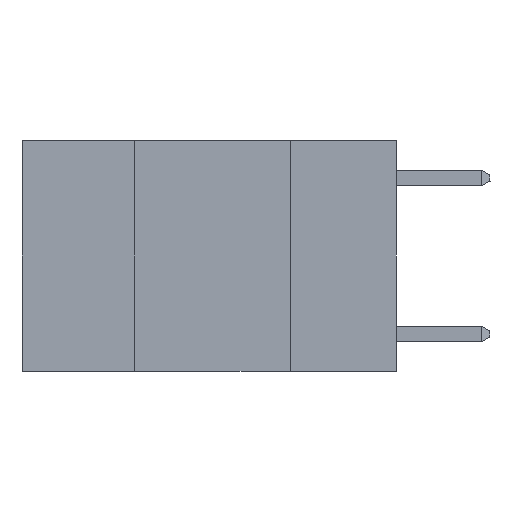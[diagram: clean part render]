
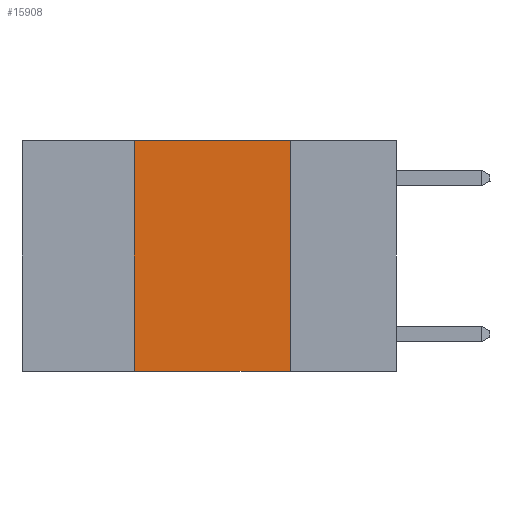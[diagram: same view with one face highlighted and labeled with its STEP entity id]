
A CAD part, left-side view. The second image highlights one B-rep face of the part: STEP entity #15908.
In plain terms, the highlighted planar face has unit normal (-1, 0, 0).
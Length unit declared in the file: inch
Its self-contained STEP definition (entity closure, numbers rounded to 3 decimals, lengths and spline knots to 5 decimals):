
#87 = CARTESIAN_POINT ( 'NONE',  ( 0., 0.42, 0. ) ) ;
#416 = LINE ( 'NONE', #87, #13189 ) ;
#472 = PLANE ( 'NONE',  #19026 ) ;
#810 = EDGE_CURVE ( 'NONE', #15724, #10061, #7259, .T. ) ;
#1289 = VECTOR ( 'NONE', #18226, 39.37008 ) ;
#1603 = CARTESIAN_POINT ( 'NONE',  ( 0., 0.6, 0. ) ) ;
#2174 = DIRECTION ( 'NONE',  ( 1., 0., 0. ) ) ;
#2742 = ORIENTED_EDGE ( 'NONE', *, *, #810, .F. ) ;
#3171 = EDGE_CURVE ( 'NONE', #3308, #10061, #6075, .T. ) ;
#3308 = VERTEX_POINT ( 'NONE', #15059 ) ;
#3775 = ORIENTED_EDGE ( 'NONE', *, *, #8630, .F. ) ;
#5020 = CARTESIAN_POINT ( 'NONE',  ( 0., 0.17, 0. ) ) ;
#5206 = LINE ( 'NONE', #1603, #1289 ) ;
#5243 = ORIENTED_EDGE ( 'NONE', *, *, #14450, .F. ) ;
#6075 = LINE ( 'NONE', #16797, #18277 ) ;
#6439 = VERTEX_POINT ( 'NONE', #8597 ) ;
#7259 = LINE ( 'NONE', #10700, #15069 ) ;
#8597 = CARTESIAN_POINT ( 'NONE',  ( 0., 0.42, 0. ) ) ;
#8630 = EDGE_CURVE ( 'NONE', #6439, #15724, #5206, .T. ) ;
#9430 = EDGE_LOOP ( 'NONE', ( #2742, #3775, #5243, #17307 ) ) ;
#10061 = VERTEX_POINT ( 'NONE', #19916 ) ;
#10700 = CARTESIAN_POINT ( 'NONE',  ( 0., 0.17, 0. ) ) ;
#10797 = DIRECTION ( 'NONE',  ( 0., 0., -1. ) ) ;
#12136 = CARTESIAN_POINT ( 'NONE',  ( 0., 0.6, 0. ) ) ;
#13189 = VECTOR ( 'NONE', #13342, 39.37008 ) ;
#13342 = DIRECTION ( 'NONE',  ( 0., 0., 1. ) ) ;
#13810 = DIRECTION ( 'NONE',  ( 0., 0., -1. ) ) ;
#14450 = EDGE_CURVE ( 'NONE', #3308, #6439, #416, .T. ) ;
#15059 = CARTESIAN_POINT ( 'NONE',  ( 0., 0.42, -0.37 ) ) ;
#15069 = VECTOR ( 'NONE', #10797, 39.37008 ) ;
#15724 = VERTEX_POINT ( 'NONE', #5020 ) ;
#15908 = ADVANCED_FACE ( 'NONE', ( #20309 ), #472, .F. ) ;
#16772 = DIRECTION ( 'NONE',  ( 0., -1., 0. ) ) ;
#16797 = CARTESIAN_POINT ( 'NONE',  ( 0., 0.6, -0.37 ) ) ;
#17307 = ORIENTED_EDGE ( 'NONE', *, *, #3171, .T. ) ;
#18226 = DIRECTION ( 'NONE',  ( 0., -1., 0. ) ) ;
#18277 = VECTOR ( 'NONE', #16772, 39.37008 ) ;
#19026 = AXIS2_PLACEMENT_3D ( 'NONE', #12136, #2174, #13810 ) ;
#19916 = CARTESIAN_POINT ( 'NONE',  ( 0., 0.17, -0.37 ) ) ;
#20309 = FACE_OUTER_BOUND ( 'NONE', #9430, .T. ) ;
